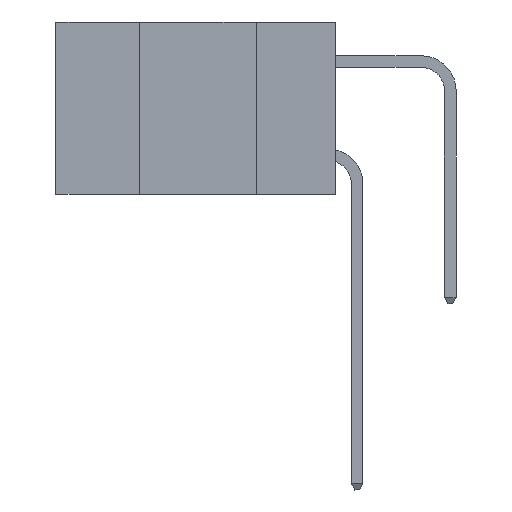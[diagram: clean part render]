
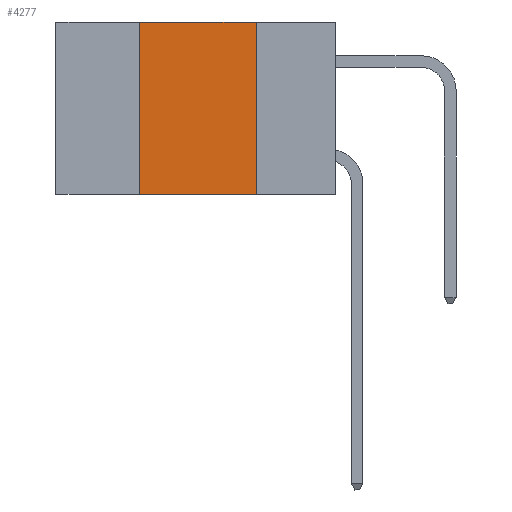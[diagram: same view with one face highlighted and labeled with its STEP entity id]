
A CAD part, left-side view. The second image highlights one B-rep face of the part: STEP entity #4277.
In plain terms, the highlighted planar face has unit normal (-1, 0, 0).
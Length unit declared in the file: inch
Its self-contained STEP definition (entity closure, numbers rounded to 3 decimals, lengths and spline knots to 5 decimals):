
#386 = VERTEX_POINT ( 'NONE', #5837 ) ;
#723 = CARTESIAN_POINT ( 'NONE',  ( 0., 0.6, 0. ) ) ;
#739 = LINE ( 'NONE', #5883, #3160 ) ;
#2404 = FACE_OUTER_BOUND ( 'NONE', #6179, .T. ) ;
#2424 = CARTESIAN_POINT ( 'NONE',  ( 0., 0.42, 0. ) ) ;
#3108 = VERTEX_POINT ( 'NONE', #13354 ) ;
#3160 = VECTOR ( 'NONE', #10976, 39.37008 ) ;
#3431 = CARTESIAN_POINT ( 'NONE',  ( 0., 0.17, -0.37 ) ) ;
#4277 = ADVANCED_FACE ( 'NONE', ( #2404 ), #7336, .F. ) ;
#4509 = VECTOR ( 'NONE', #13388, 39.37008 ) ;
#5166 = VERTEX_POINT ( 'NONE', #3431 ) ;
#5174 = DIRECTION ( 'NONE',  ( 0., 0., -1. ) ) ;
#5615 = LINE ( 'NONE', #723, #8061 ) ;
#5814 = ORIENTED_EDGE ( 'NONE', *, *, #8352, .F. ) ;
#5837 = CARTESIAN_POINT ( 'NONE',  ( 0., 0.42, 0. ) ) ;
#5883 = CARTESIAN_POINT ( 'NONE',  ( 0., 0.17, 0. ) ) ;
#6043 = VERTEX_POINT ( 'NONE', #13542 ) ;
#6179 = EDGE_LOOP ( 'NONE', ( #13327, #5814, #9022, #11075 ) ) ;
#6295 = LINE ( 'NONE', #2424, #9012 ) ;
#6304 = CARTESIAN_POINT ( 'NONE',  ( 0., 0.6, -0.37 ) ) ;
#7336 = PLANE ( 'NONE',  #12484 ) ;
#7544 = CARTESIAN_POINT ( 'NONE',  ( 0., 0.6, 0. ) ) ;
#7561 = DIRECTION ( 'NONE',  ( 1., 0., 0. ) ) ;
#7834 = DIRECTION ( 'NONE',  ( 0., 0., 1. ) ) ;
#8061 = VECTOR ( 'NONE', #9476, 39.37008 ) ;
#8352 = EDGE_CURVE ( 'NONE', #386, #3108, #5615, .T. ) ;
#9012 = VECTOR ( 'NONE', #7834, 39.37008 ) ;
#9022 = ORIENTED_EDGE ( 'NONE', *, *, #10327, .F. ) ;
#9476 = DIRECTION ( 'NONE',  ( 0., -1., 0. ) ) ;
#10327 = EDGE_CURVE ( 'NONE', #6043, #386, #6295, .T. ) ;
#10976 = DIRECTION ( 'NONE',  ( 0., 0., -1. ) ) ;
#11012 = EDGE_CURVE ( 'NONE', #3108, #5166, #739, .T. ) ;
#11075 = ORIENTED_EDGE ( 'NONE', *, *, #13060, .T. ) ;
#12484 = AXIS2_PLACEMENT_3D ( 'NONE', #7544, #7561, #5174 ) ;
#13060 = EDGE_CURVE ( 'NONE', #6043, #5166, #13062, .T. ) ;
#13062 = LINE ( 'NONE', #6304, #4509 ) ;
#13327 = ORIENTED_EDGE ( 'NONE', *, *, #11012, .F. ) ;
#13354 = CARTESIAN_POINT ( 'NONE',  ( 0., 0.17, 0. ) ) ;
#13388 = DIRECTION ( 'NONE',  ( 0., -1., 0. ) ) ;
#13542 = CARTESIAN_POINT ( 'NONE',  ( 0., 0.42, -0.37 ) ) ;
